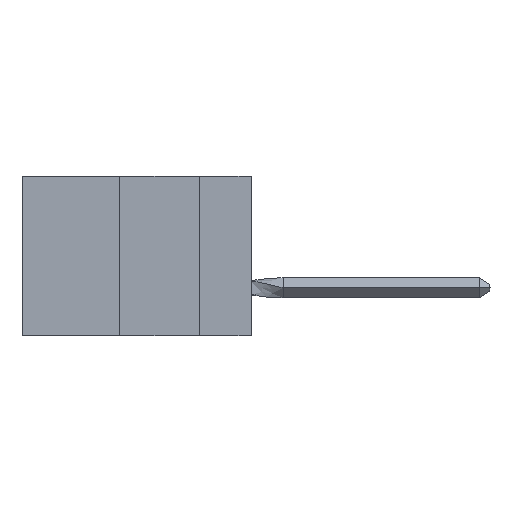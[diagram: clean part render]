
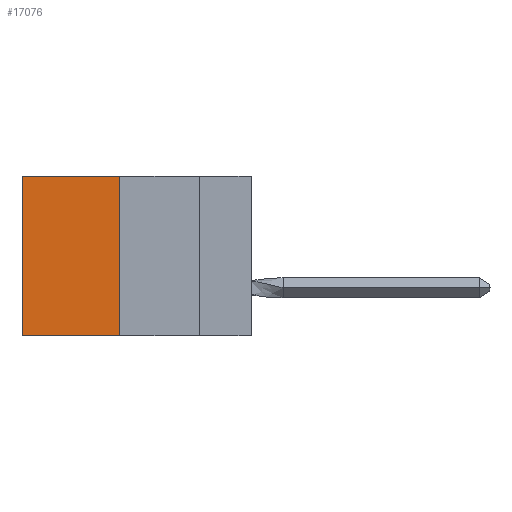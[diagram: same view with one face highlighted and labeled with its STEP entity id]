
A CAD part, left-side view. The second image highlights one B-rep face of the part: STEP entity #17076.
In plain terms, the highlighted planar face has unit normal (-1, 0, 0).
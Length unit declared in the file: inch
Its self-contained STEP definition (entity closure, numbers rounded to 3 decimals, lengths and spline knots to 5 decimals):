
#1322 = VERTEX_POINT ( 'NONE', #23450 ) ;
#2464 = CARTESIAN_POINT ( 'NONE',  ( 0.305, 0.72, -0.5 ) ) ;
#3112 = VECTOR ( 'NONE', #19010, 39.37008 ) ;
#3586 = EDGE_LOOP ( 'NONE', ( #10839, #15702, #17238, #11404 ) ) ;
#3823 = LINE ( 'NONE', #15256, #11417 ) ;
#3959 = EDGE_CURVE ( 'NONE', #9678, #5535, #10119, .T. ) ;
#5096 = DIRECTION ( 'NONE',  ( 1., 0., 0. ) ) ;
#5535 = VERTEX_POINT ( 'NONE', #7069 ) ;
#5873 = EDGE_CURVE ( 'NONE', #9678, #1322, #19145, .T. ) ;
#5931 = DIRECTION ( 'NONE',  ( 0., 1., 0. ) ) ;
#6029 = CARTESIAN_POINT ( 'NONE',  ( 0.305, 0.72, -0.5 ) ) ;
#6088 = CARTESIAN_POINT ( 'NONE',  ( 0.305, 0.413, 0. ) ) ;
#6380 = DIRECTION ( 'NONE',  ( 0., 0., -1. ) ) ;
#6971 = CARTESIAN_POINT ( 'NONE',  ( 0.305, 0.413, -0.5 ) ) ;
#7069 = CARTESIAN_POINT ( 'NONE',  ( 0.305, 0.413, -0.5 ) ) ;
#8065 = DIRECTION ( 'NONE',  ( 0., 1., 0. ) ) ;
#9084 = CARTESIAN_POINT ( 'NONE',  ( 0.305, 0.413, -0.5 ) ) ;
#9678 = VERTEX_POINT ( 'NONE', #12082 ) ;
#10119 = LINE ( 'NONE', #9084, #3112 ) ;
#10839 = ORIENTED_EDGE ( 'NONE', *, *, #18349, .T. ) ;
#11404 = ORIENTED_EDGE ( 'NONE', *, *, #5873, .T. ) ;
#11417 = VECTOR ( 'NONE', #5931, 39.37008 ) ;
#12082 = CARTESIAN_POINT ( 'NONE',  ( 0.305, 0.413, 0. ) ) ;
#15256 = CARTESIAN_POINT ( 'NONE',  ( 0.305, 0.413, -0.5 ) ) ;
#15479 = EDGE_CURVE ( 'NONE', #5535, #23139, #3823, .T. ) ;
#15702 = ORIENTED_EDGE ( 'NONE', *, *, #15479, .F. ) ;
#17076 = ADVANCED_FACE ( 'NONE', ( #19532 ), #18596, .F. ) ;
#17238 = ORIENTED_EDGE ( 'NONE', *, *, #3959, .F. ) ;
#18349 = EDGE_CURVE ( 'NONE', #1322, #23139, #19159, .T. ) ;
#18596 = PLANE ( 'NONE',  #21621 ) ;
#19010 = DIRECTION ( 'NONE',  ( 0., 0., -1. ) ) ;
#19145 = LINE ( 'NONE', #6088, #21866 ) ;
#19159 = LINE ( 'NONE', #2464, #19747 ) ;
#19532 = FACE_OUTER_BOUND ( 'NONE', #3586, .T. ) ;
#19747 = VECTOR ( 'NONE', #6380, 39.37008 ) ;
#21621 = AXIS2_PLACEMENT_3D ( 'NONE', #6971, #5096, #22510 ) ;
#21866 = VECTOR ( 'NONE', #8065, 39.37008 ) ;
#22510 = DIRECTION ( 'NONE',  ( 0., 0., -1. ) ) ;
#23139 = VERTEX_POINT ( 'NONE', #6029 ) ;
#23450 = CARTESIAN_POINT ( 'NONE',  ( 0.305, 0.72, 0. ) ) ;
